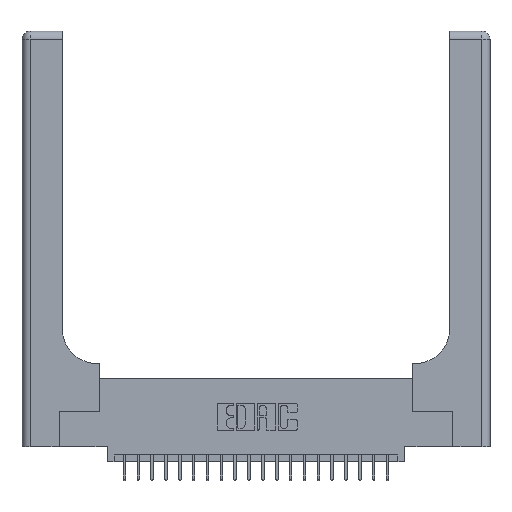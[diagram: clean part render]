
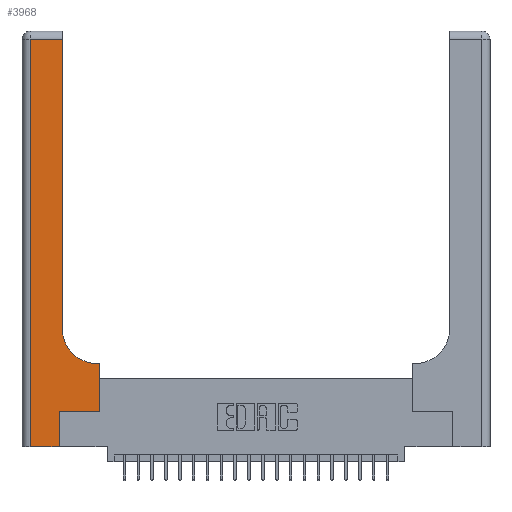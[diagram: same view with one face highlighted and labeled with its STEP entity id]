
A CAD part, top view. The second image highlights one B-rep face of the part: STEP entity #3968.
In plain terms, the highlighted planar face has unit normal (0, 0, 1).
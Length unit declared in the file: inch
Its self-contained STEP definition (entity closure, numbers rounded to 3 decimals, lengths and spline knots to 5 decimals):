
#145 = DIRECTION ( 'NONE',  ( 0., -1., 0. ) ) ;
#727 = ORIENTED_EDGE ( 'NONE', *, *, #13453, .T. ) ;
#969 = EDGE_CURVE ( 'NONE', #13831, #11868, #17607, .T. ) ;
#1147 = CARTESIAN_POINT ( 'NONE',  ( 0., 3., 0.37 ) ) ;
#1187 = EDGE_CURVE ( 'NONE', #11868, #13730, #18207, .T. ) ;
#1263 = LINE ( 'NONE', #11984, #22380 ) ;
#2448 = LINE ( 'NONE', #16851, #23733 ) ;
#2583 = VERTEX_POINT ( 'NONE', #17127 ) ;
#2772 = EDGE_LOOP ( 'NONE', ( #15081, #12286, #5669, #18521, #17304, #7968, #13446, #727, #20550 ) ) ;
#2810 = CARTESIAN_POINT ( 'NONE',  ( 0.06, 0., 0.37 ) ) ;
#2983 = FACE_OUTER_BOUND ( 'NONE', #2772, .T. ) ;
#3451 = DIRECTION ( 'NONE',  ( 0., 1., 0. ) ) ;
#3679 = AXIS2_PLACEMENT_3D ( 'NONE', #16957, #9374, #18666 ) ;
#3880 = EDGE_CURVE ( 'NONE', #14206, #6480, #1263, .T. ) ;
#3906 = VECTOR ( 'NONE', #21672, 39.37008 ) ;
#3968 = ADVANCED_FACE ( 'NONE', ( #2983 ), #23439, .F. ) ;
#4094 = VECTOR ( 'NONE', #5162, 39.37008 ) ;
#4436 = CARTESIAN_POINT ( 'NONE',  ( 0.269, 0.25, 0.37 ) ) ;
#4548 = LINE ( 'NONE', #11978, #18109 ) ;
#4670 = CARTESIAN_POINT ( 'NONE',  ( 0.269, 0.25, 0.37 ) ) ;
#4916 = CARTESIAN_POINT ( 'NONE',  ( 0.5585, 0.6, 0.37 ) ) ;
#5054 = CARTESIAN_POINT ( 'NONE',  ( 0.5415, 0.6, 0.37 ) ) ;
#5162 = DIRECTION ( 'NONE',  ( 0., 1., 0. ) ) ;
#5669 = ORIENTED_EDGE ( 'NONE', *, *, #14150, .T. ) ;
#6480 = VERTEX_POINT ( 'NONE', #6980 ) ;
#6640 = LINE ( 'NONE', #19705, #4094 ) ;
#6722 = EDGE_CURVE ( 'NONE', #14825, #19480, #20324, .T. ) ;
#6980 = CARTESIAN_POINT ( 'NONE',  ( 0.269, 0., 0.37 ) ) ;
#7378 = CARTESIAN_POINT ( 'NONE',  ( 0.06, 2.94, 0.37 ) ) ;
#7601 = DIRECTION ( 'NONE',  ( -1., 0., 0. ) ) ;
#7627 = DIRECTION ( 'NONE',  ( 1., 0., 0. ) ) ;
#7860 = VECTOR ( 'NONE', #7627, 39.37008 ) ;
#7968 = ORIENTED_EDGE ( 'NONE', *, *, #969, .T. ) ;
#8562 = DIRECTION ( 'NONE',  ( 0., 0., -1. ) ) ;
#9374 = DIRECTION ( 'NONE',  ( 0., 0., -1. ) ) ;
#10700 = AXIS2_PLACEMENT_3D ( 'NONE', #1147, #8562, #21622 ) ;
#11868 = VERTEX_POINT ( 'NONE', #17030 ) ;
#11978 = CARTESIAN_POINT ( 'NONE',  ( 0.2915, 3., 0.37 ) ) ;
#11984 = CARTESIAN_POINT ( 'NONE',  ( 0., 0., 0.37 ) ) ;
#12286 = ORIENTED_EDGE ( 'NONE', *, *, #6722, .T. ) ;
#12588 = CARTESIAN_POINT ( 'NONE',  ( 0.5585, 0.25, 0.37 ) ) ;
#13446 = ORIENTED_EDGE ( 'NONE', *, *, #1187, .T. ) ;
#13453 = EDGE_CURVE ( 'NONE', #13730, #18324, #17900, .T. ) ;
#13730 = VERTEX_POINT ( 'NONE', #4916 ) ;
#13764 = VECTOR ( 'NONE', #3451, 39.37008 ) ;
#13831 = VERTEX_POINT ( 'NONE', #4670 ) ;
#14150 = EDGE_CURVE ( 'NONE', #19480, #14206, #2448, .T. ) ;
#14206 = VERTEX_POINT ( 'NONE', #2810 ) ;
#14825 = VERTEX_POINT ( 'NONE', #24007 ) ;
#15081 = ORIENTED_EDGE ( 'NONE', *, *, #18782, .T. ) ;
#16018 = EDGE_CURVE ( 'NONE', #18324, #2583, #16531, .T. ) ;
#16036 = DIRECTION ( 'NONE',  ( 1., 0., 0. ) ) ;
#16531 = CIRCLE ( 'NONE', #3679, 0.25 ) ;
#16599 = VECTOR ( 'NONE', #7601, 39.37008 ) ;
#16851 = CARTESIAN_POINT ( 'NONE',  ( 0.06, 3., 0.37 ) ) ;
#16957 = CARTESIAN_POINT ( 'NONE',  ( 0.5415, 0.85, 0.37 ) ) ;
#17030 = CARTESIAN_POINT ( 'NONE',  ( 0.5585, 0.25, 0.37 ) ) ;
#17127 = CARTESIAN_POINT ( 'NONE',  ( 0.2915, 0.85, 0.37 ) ) ;
#17224 = EDGE_CURVE ( 'NONE', #6480, #13831, #6640, .T. ) ;
#17304 = ORIENTED_EDGE ( 'NONE', *, *, #17224, .T. ) ;
#17607 = LINE ( 'NONE', #4436, #7860 ) ;
#17900 = LINE ( 'NONE', #23482, #3906 ) ;
#18109 = VECTOR ( 'NONE', #19437, 39.37008 ) ;
#18207 = LINE ( 'NONE', #12588, #13764 ) ;
#18324 = VERTEX_POINT ( 'NONE', #5054 ) ;
#18521 = ORIENTED_EDGE ( 'NONE', *, *, #3880, .T. ) ;
#18666 = DIRECTION ( 'NONE',  ( 1., 0., 0. ) ) ;
#18782 = EDGE_CURVE ( 'NONE', #2583, #14825, #4548, .T. ) ;
#19437 = DIRECTION ( 'NONE',  ( 0., 1., 0. ) ) ;
#19480 = VERTEX_POINT ( 'NONE', #7378 ) ;
#19705 = CARTESIAN_POINT ( 'NONE',  ( 0.269, 0., 0.37 ) ) ;
#20324 = LINE ( 'NONE', #23953, #16599 ) ;
#20550 = ORIENTED_EDGE ( 'NONE', *, *, #16018, .T. ) ;
#21622 = DIRECTION ( 'NONE',  ( -1., 0., 0. ) ) ;
#21672 = DIRECTION ( 'NONE',  ( -1., 0., 0. ) ) ;
#22380 = VECTOR ( 'NONE', #16036, 39.37008 ) ;
#23439 = PLANE ( 'NONE',  #10700 ) ;
#23482 = CARTESIAN_POINT ( 'NONE',  ( 0.2915, 0.6, 0.37 ) ) ;
#23733 = VECTOR ( 'NONE', #145, 39.37008 ) ;
#23953 = CARTESIAN_POINT ( 'NONE',  ( 0., 2.94, 0.37 ) ) ;
#24007 = CARTESIAN_POINT ( 'NONE',  ( 0.2915, 2.94, 0.37 ) ) ;
